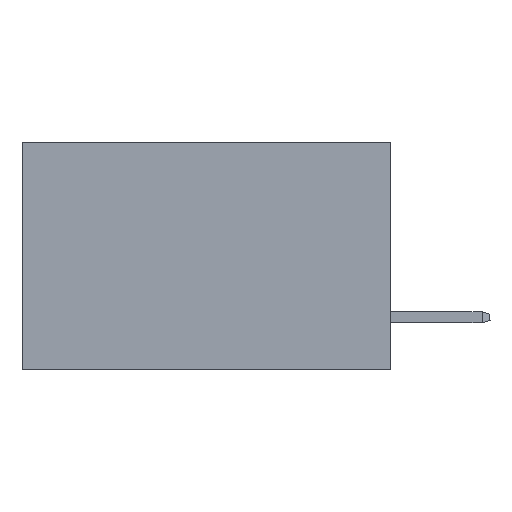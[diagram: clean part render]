
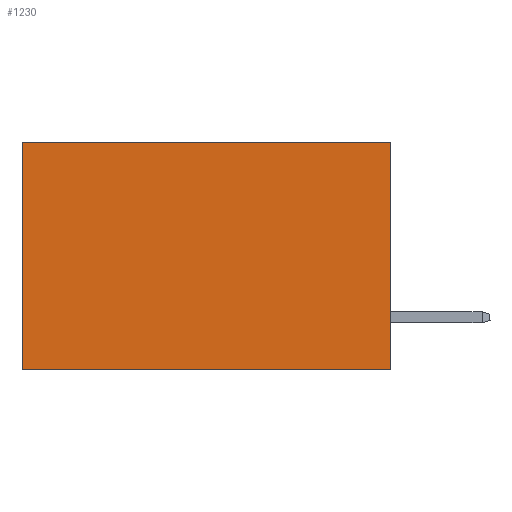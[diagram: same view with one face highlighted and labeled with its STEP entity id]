
A CAD part, left-side view. The second image highlights one B-rep face of the part: STEP entity #1230.
In plain terms, the highlighted planar face has unit normal (-1, 0, 0).
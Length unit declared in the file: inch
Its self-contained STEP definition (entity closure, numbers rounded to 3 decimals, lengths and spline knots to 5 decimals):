
#455 = CARTESIAN_POINT ( 'NONE',  ( 0.2875, 0., 0. ) ) ;
#1230 = ADVANCED_FACE ( 'NONE', ( #16689 ), #14452, .F. ) ;
#1921 = LINE ( 'NONE', #455, #4034 ) ;
#2319 = AXIS2_PLACEMENT_3D ( 'NONE', #19561, #3269, #33762 ) ;
#2570 = CARTESIAN_POINT ( 'NONE',  ( 0.2875, 0.6, -0.37 ) ) ;
#3269 = DIRECTION ( 'NONE',  ( 1., 0., 0. ) ) ;
#3866 = VECTOR ( 'NONE', #4441, 39.37008 ) ;
#3970 = CARTESIAN_POINT ( 'NONE',  ( 0.2875, 0., 0. ) ) ;
#4034 = VECTOR ( 'NONE', #32130, 39.37008 ) ;
#4293 = LINE ( 'NONE', #3970, #32771 ) ;
#4298 = VERTEX_POINT ( 'NONE', #6116 ) ;
#4441 = DIRECTION ( 'NONE',  ( 0., 0., -1. ) ) ;
#5118 = ORIENTED_EDGE ( 'NONE', *, *, #26320, .F. ) ;
#5964 = EDGE_CURVE ( 'NONE', #10681, #4298, #4293, .T. ) ;
#6116 = CARTESIAN_POINT ( 'NONE',  ( 0.2875, 0., -0.37 ) ) ;
#6992 = CARTESIAN_POINT ( 'NONE',  ( 0.2875, 0.6, 0. ) ) ;
#10496 = VERTEX_POINT ( 'NONE', #6992 ) ;
#10681 = VERTEX_POINT ( 'NONE', #29359 ) ;
#11672 = EDGE_LOOP ( 'NONE', ( #25723, #5118, #28048, #19081 ) ) ;
#12179 = LINE ( 'NONE', #17622, #28561 ) ;
#12984 = CARTESIAN_POINT ( 'NONE',  ( 0.2875, 0.6, 0. ) ) ;
#14452 = PLANE ( 'NONE',  #2319 ) ;
#16689 = FACE_OUTER_BOUND ( 'NONE', #11672, .T. ) ;
#17622 = CARTESIAN_POINT ( 'NONE',  ( 0.2875, 0., -0.37 ) ) ;
#19081 = ORIENTED_EDGE ( 'NONE', *, *, #22279, .T. ) ;
#19561 = CARTESIAN_POINT ( 'NONE',  ( 0.2875, 0., 0. ) ) ;
#20534 = DIRECTION ( 'NONE',  ( 0., 1., 0. ) ) ;
#22279 = EDGE_CURVE ( 'NONE', #10681, #10496, #1921, .T. ) ;
#24632 = LINE ( 'NONE', #12984, #3866 ) ;
#25723 = ORIENTED_EDGE ( 'NONE', *, *, #35089, .T. ) ;
#26320 = EDGE_CURVE ( 'NONE', #4298, #30446, #12179, .T. ) ;
#28048 = ORIENTED_EDGE ( 'NONE', *, *, #5964, .F. ) ;
#28541 = DIRECTION ( 'NONE',  ( 0., 0., -1. ) ) ;
#28561 = VECTOR ( 'NONE', #20534, 39.37008 ) ;
#29359 = CARTESIAN_POINT ( 'NONE',  ( 0.2875, 0., 0. ) ) ;
#30446 = VERTEX_POINT ( 'NONE', #2570 ) ;
#32130 = DIRECTION ( 'NONE',  ( 0., 1., 0. ) ) ;
#32771 = VECTOR ( 'NONE', #28541, 39.37008 ) ;
#33762 = DIRECTION ( 'NONE',  ( 0., 0., -1. ) ) ;
#35089 = EDGE_CURVE ( 'NONE', #10496, #30446, #24632, .T. ) ;
